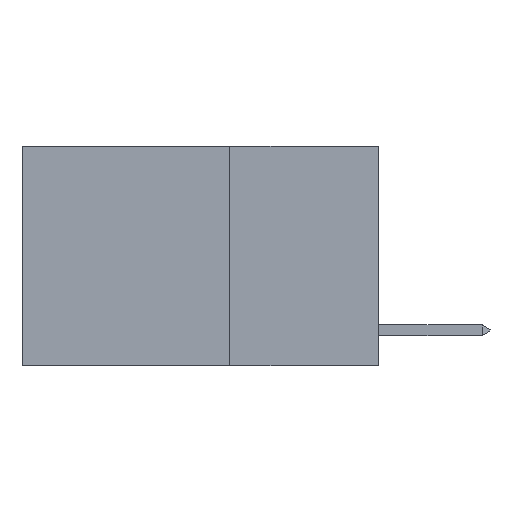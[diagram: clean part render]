
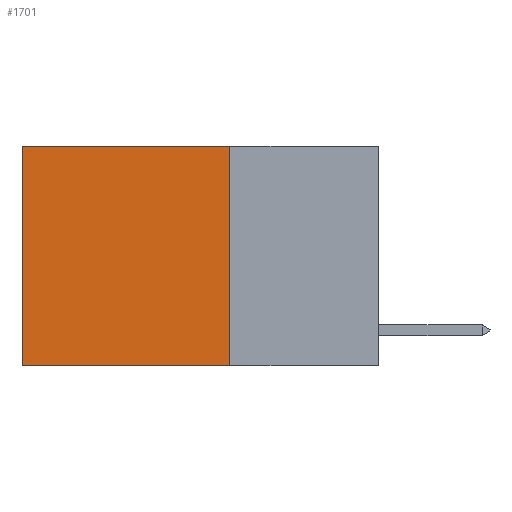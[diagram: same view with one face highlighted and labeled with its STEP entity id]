
A CAD part, left-side view. The second image highlights one B-rep face of the part: STEP entity #1701.
In plain terms, the highlighted planar face has unit normal (-1, 0, 0).
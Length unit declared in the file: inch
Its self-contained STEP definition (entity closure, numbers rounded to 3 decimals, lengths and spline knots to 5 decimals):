
#1280 = CARTESIAN_POINT ( 'NONE',  ( 0.2625, 0.25, 0. ) ) ;
#1701 = ADVANCED_FACE ( 'NONE', ( #20246 ), #1914, .F. ) ;
#1914 = PLANE ( 'NONE',  #23740 ) ;
#2280 = DIRECTION ( 'NONE',  ( 0., 1., 0. ) ) ;
#3195 = CARTESIAN_POINT ( 'NONE',  ( 0.2625, 0.25, 0. ) ) ;
#4901 = ORIENTED_EDGE ( 'NONE', *, *, #14362, .F. ) ;
#5641 = ORIENTED_EDGE ( 'NONE', *, *, #10214, .F. ) ;
#6408 = DIRECTION ( 'NONE',  ( 0., 0., -1. ) ) ;
#6774 = CARTESIAN_POINT ( 'NONE',  ( 0.2625, 0.25, -0.37 ) ) ;
#7767 = VERTEX_POINT ( 'NONE', #24175 ) ;
#7876 = EDGE_CURVE ( 'NONE', #21571, #23545, #25953, .T. ) ;
#8307 = VECTOR ( 'NONE', #26256, 39.37008 ) ;
#9036 = CARTESIAN_POINT ( 'NONE',  ( 0.2625, 0.25, 0. ) ) ;
#10214 = EDGE_CURVE ( 'NONE', #23031, #7767, #14129, .T. ) ;
#11526 = CARTESIAN_POINT ( 'NONE',  ( 0.2625, 0.6, 0. ) ) ;
#13298 = ORIENTED_EDGE ( 'NONE', *, *, #7876, .T. ) ;
#14129 = LINE ( 'NONE', #9036, #8307 ) ;
#14362 = EDGE_CURVE ( 'NONE', #7767, #23545, #24962, .T. ) ;
#14622 = VECTOR ( 'NONE', #20298, 39.37008 ) ;
#16058 = CARTESIAN_POINT ( 'NONE',  ( 0.2625, 0.6, 0. ) ) ;
#17283 = CARTESIAN_POINT ( 'NONE',  ( 0.2625, 0.25, 0. ) ) ;
#17743 = VECTOR ( 'NONE', #20675, 39.37008 ) ;
#17865 = EDGE_LOOP ( 'NONE', ( #13298, #4901, #5641, #27584 ) ) ;
#19466 = DIRECTION ( 'NONE',  ( 1., 0., 0. ) ) ;
#19998 = EDGE_CURVE ( 'NONE', #23031, #21571, #27724, .T. ) ;
#20007 = VECTOR ( 'NONE', #2280, 39.37008 ) ;
#20246 = FACE_OUTER_BOUND ( 'NONE', #17865, .T. ) ;
#20298 = DIRECTION ( 'NONE',  ( 0., 0., -1. ) ) ;
#20675 = DIRECTION ( 'NONE',  ( 0., 1., 0. ) ) ;
#21571 = VERTEX_POINT ( 'NONE', #16058 ) ;
#23031 = VERTEX_POINT ( 'NONE', #1280 ) ;
#23545 = VERTEX_POINT ( 'NONE', #24827 ) ;
#23740 = AXIS2_PLACEMENT_3D ( 'NONE', #17283, #19466, #6408 ) ;
#24175 = CARTESIAN_POINT ( 'NONE',  ( 0.2625, 0.25, -0.37 ) ) ;
#24827 = CARTESIAN_POINT ( 'NONE',  ( 0.2625, 0.6, -0.37 ) ) ;
#24962 = LINE ( 'NONE', #6774, #20007 ) ;
#25953 = LINE ( 'NONE', #11526, #14622 ) ;
#26256 = DIRECTION ( 'NONE',  ( 0., 0., -1. ) ) ;
#27584 = ORIENTED_EDGE ( 'NONE', *, *, #19998, .T. ) ;
#27724 = LINE ( 'NONE', #3195, #17743 ) ;
